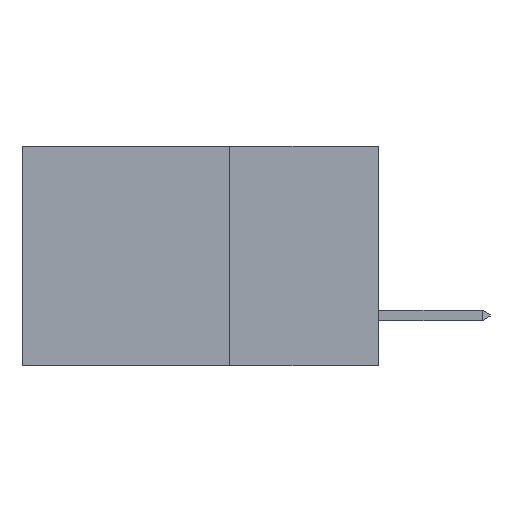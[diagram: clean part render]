
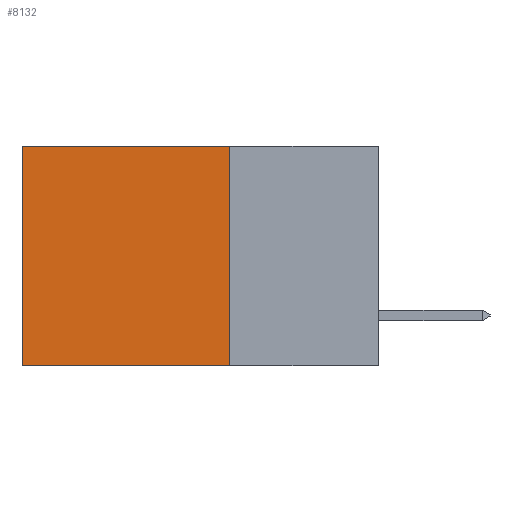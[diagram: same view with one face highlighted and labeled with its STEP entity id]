
A CAD part, left-side view. The second image highlights one B-rep face of the part: STEP entity #8132.
In plain terms, the highlighted planar face has unit normal (-1, 0, 0).
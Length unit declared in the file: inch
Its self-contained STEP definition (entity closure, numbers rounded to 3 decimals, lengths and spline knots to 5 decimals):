
#492 = CARTESIAN_POINT ( 'NONE',  ( 0.2615, 0.6, -0.37 ) ) ;
#1738 = ORIENTED_EDGE ( 'NONE', *, *, #19289, .T. ) ;
#1822 = VECTOR ( 'NONE', #20555, 39.37008 ) ;
#1914 = VERTEX_POINT ( 'NONE', #20061 ) ;
#1919 = LINE ( 'NONE', #4417, #16575 ) ;
#3360 = EDGE_CURVE ( 'NONE', #1914, #10453, #1919, .T. ) ;
#3436 = FACE_OUTER_BOUND ( 'NONE', #17137, .T. ) ;
#4222 = AXIS2_PLACEMENT_3D ( 'NONE', #16211, #16017, #15968 ) ;
#4413 = DIRECTION ( 'NONE',  ( 0., 0., -1. ) ) ;
#4417 = CARTESIAN_POINT ( 'NONE',  ( 0.2615, 0.25, -0.37 ) ) ;
#5238 = EDGE_CURVE ( 'NONE', #10453, #9096, #6358, .T. ) ;
#5561 = ORIENTED_EDGE ( 'NONE', *, *, #11589, .T. ) ;
#6358 = LINE ( 'NONE', #12793, #20458 ) ;
#8036 = CARTESIAN_POINT ( 'NONE',  ( 0.2615, 0.6, 0. ) ) ;
#8132 = ADVANCED_FACE ( 'NONE', ( #3436 ), #16121, .F. ) ;
#8975 = CARTESIAN_POINT ( 'NONE',  ( 0.2615, 0.6, -0.37 ) ) ;
#9096 = VERTEX_POINT ( 'NONE', #8975 ) ;
#9750 = ORIENTED_EDGE ( 'NONE', *, *, #5238, .F. ) ;
#9870 = DIRECTION ( 'NONE',  ( 0., 1., 0. ) ) ;
#10080 = CARTESIAN_POINT ( 'NONE',  ( 0.2615, 0.25, 0. ) ) ;
#10453 = VERTEX_POINT ( 'NONE', #18559 ) ;
#10710 = DIRECTION ( 'NONE',  ( 0., 1., 0. ) ) ;
#11589 = EDGE_CURVE ( 'NONE', #1914, #22822, #23552, .T. ) ;
#12793 = CARTESIAN_POINT ( 'NONE',  ( 0.2615, 0.25, -0.37 ) ) ;
#13908 = VECTOR ( 'NONE', #9870, 39.37008 ) ;
#15968 = DIRECTION ( 'NONE',  ( 0., 0., -1. ) ) ;
#16017 = DIRECTION ( 'NONE',  ( 1., 0., 0. ) ) ;
#16121 = PLANE ( 'NONE',  #4222 ) ;
#16211 = CARTESIAN_POINT ( 'NONE',  ( 0.2615, 0.25, -0.37 ) ) ;
#16482 = LINE ( 'NONE', #492, #1822 ) ;
#16575 = VECTOR ( 'NONE', #4413, 39.37008 ) ;
#17137 = EDGE_LOOP ( 'NONE', ( #1738, #9750, #20198, #5561 ) ) ;
#18559 = CARTESIAN_POINT ( 'NONE',  ( 0.2615, 0.25, -0.37 ) ) ;
#19289 = EDGE_CURVE ( 'NONE', #22822, #9096, #16482, .T. ) ;
#20061 = CARTESIAN_POINT ( 'NONE',  ( 0.2615, 0.25, 0. ) ) ;
#20198 = ORIENTED_EDGE ( 'NONE', *, *, #3360, .F. ) ;
#20458 = VECTOR ( 'NONE', #10710, 39.37008 ) ;
#20555 = DIRECTION ( 'NONE',  ( 0., 0., -1. ) ) ;
#22822 = VERTEX_POINT ( 'NONE', #8036 ) ;
#23552 = LINE ( 'NONE', #10080, #13908 ) ;
